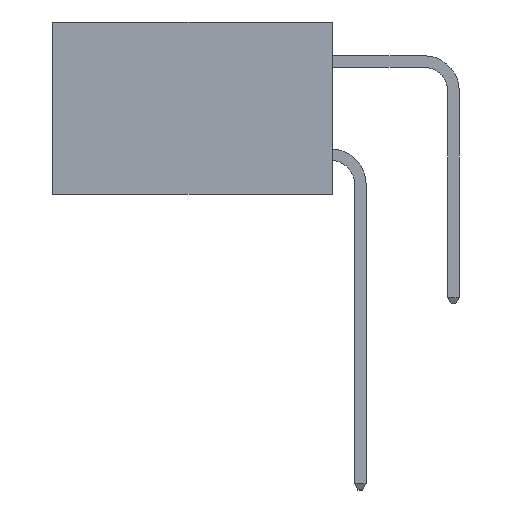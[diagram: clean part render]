
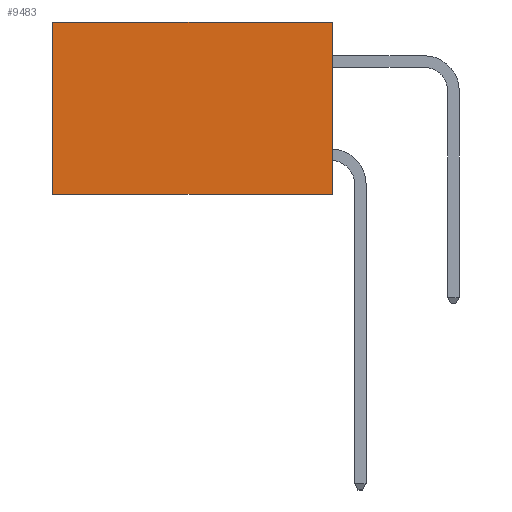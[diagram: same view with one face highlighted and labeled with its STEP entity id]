
A CAD part, left-side view. The second image highlights one B-rep face of the part: STEP entity #9483.
In plain terms, the highlighted planar face has unit normal (-1, 0, 0).
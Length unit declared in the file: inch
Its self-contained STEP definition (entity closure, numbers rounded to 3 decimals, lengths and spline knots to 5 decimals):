
#424 = CARTESIAN_POINT ( 'NONE',  ( 0.2615, 0., -0.37 ) ) ;
#514 = VECTOR ( 'NONE', #2638, 39.37008 ) ;
#866 = VECTOR ( 'NONE', #7317, 39.37008 ) ;
#1693 = CARTESIAN_POINT ( 'NONE',  ( 0.2615, 0., -0.37 ) ) ;
#1725 = VERTEX_POINT ( 'NONE', #7867 ) ;
#2491 = VERTEX_POINT ( 'NONE', #8630 ) ;
#2638 = DIRECTION ( 'NONE',  ( 0., 1., 0. ) ) ;
#2761 = CARTESIAN_POINT ( 'NONE',  ( 0.2615, 0., 0. ) ) ;
#3009 = EDGE_CURVE ( 'NONE', #1725, #2491, #10800, .T. ) ;
#3119 = ORIENTED_EDGE ( 'NONE', *, *, #9917, .F. ) ;
#3131 = ORIENTED_EDGE ( 'NONE', *, *, #9212, .T. ) ;
#3223 = ORIENTED_EDGE ( 'NONE', *, *, #5443, .F. ) ;
#3474 = DIRECTION ( 'NONE',  ( 0., 1., 0. ) ) ;
#3506 = ORIENTED_EDGE ( 'NONE', *, *, #3009, .T. ) ;
#3584 = LINE ( 'NONE', #6412, #866 ) ;
#4884 = PLANE ( 'NONE',  #8017 ) ;
#5119 = LINE ( 'NONE', #11146, #11957 ) ;
#5443 = EDGE_CURVE ( 'NONE', #1725, #6884, #5119, .T. ) ;
#5638 = CARTESIAN_POINT ( 'NONE',  ( 0.2615, 0.6, -0.37 ) ) ;
#5780 = DIRECTION ( 'NONE',  ( 0., 0., -1. ) ) ;
#5786 = DIRECTION ( 'NONE',  ( 0., 0., -1. ) ) ;
#5899 = LINE ( 'NONE', #424, #10405 ) ;
#6412 = CARTESIAN_POINT ( 'NONE',  ( 0.2615, 0.6, -0.37 ) ) ;
#6884 = VERTEX_POINT ( 'NONE', #1693 ) ;
#6946 = VERTEX_POINT ( 'NONE', #5638 ) ;
#7317 = DIRECTION ( 'NONE',  ( 0., 0., -1. ) ) ;
#7867 = CARTESIAN_POINT ( 'NONE',  ( 0.2615, 0., 0. ) ) ;
#8017 = AXIS2_PLACEMENT_3D ( 'NONE', #10280, #11156, #5786 ) ;
#8630 = CARTESIAN_POINT ( 'NONE',  ( 0.2615, 0.6, 0. ) ) ;
#9212 = EDGE_CURVE ( 'NONE', #2491, #6946, #3584, .T. ) ;
#9483 = ADVANCED_FACE ( 'NONE', ( #11210 ), #4884, .F. ) ;
#9917 = EDGE_CURVE ( 'NONE', #6884, #6946, #5899, .T. ) ;
#10280 = CARTESIAN_POINT ( 'NONE',  ( 0.2615, 0., -0.37 ) ) ;
#10405 = VECTOR ( 'NONE', #3474, 39.37008 ) ;
#10800 = LINE ( 'NONE', #2761, #514 ) ;
#11146 = CARTESIAN_POINT ( 'NONE',  ( 0.2615, 0., -0.37 ) ) ;
#11156 = DIRECTION ( 'NONE',  ( 1., 0., 0. ) ) ;
#11210 = FACE_OUTER_BOUND ( 'NONE', #11966, .T. ) ;
#11957 = VECTOR ( 'NONE', #5780, 39.37008 ) ;
#11966 = EDGE_LOOP ( 'NONE', ( #3131, #3119, #3223, #3506 ) ) ;
